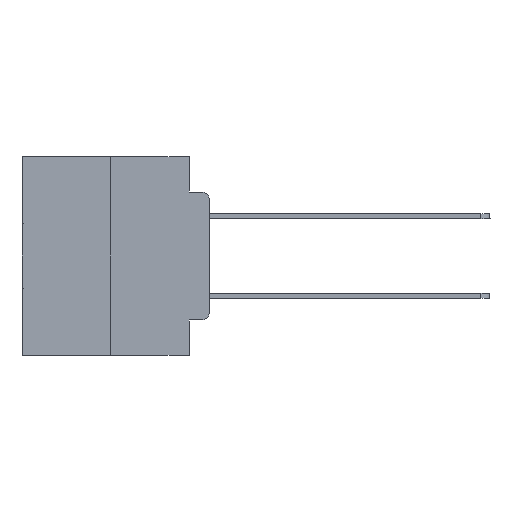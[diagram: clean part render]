
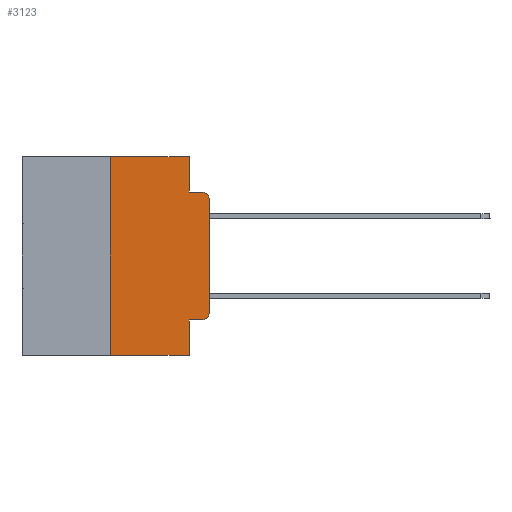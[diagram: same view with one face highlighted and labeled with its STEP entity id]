
A CAD part, left-side view. The second image highlights one B-rep face of the part: STEP entity #3123.
In plain terms, the highlighted planar face has unit normal (-1, 0, 0).
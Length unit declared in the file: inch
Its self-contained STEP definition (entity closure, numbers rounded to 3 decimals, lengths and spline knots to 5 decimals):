
#563 = ORIENTED_EDGE ( 'NONE', *, *, #14449, .T. ) ;
#740 = CARTESIAN_POINT ( 'NONE',  ( 0., 0.25, 0. ) ) ;
#983 = DIRECTION ( 'NONE',  ( 0., 0., -1. ) ) ;
#1638 = CARTESIAN_POINT ( 'NONE',  ( 0., 0.25, 0. ) ) ;
#3033 = LINE ( 'NONE', #27077, #23348 ) ;
#3123 = ADVANCED_FACE ( 'NONE', ( #18397 ), #16786, .F. ) ;
#3356 = CARTESIAN_POINT ( 'NONE',  ( 0., 0.051, -0.0885 ) ) ;
#3423 = CARTESIAN_POINT ( 'NONE',  ( 0., 0.02, -0.3915 ) ) ;
#3511 = DIRECTION ( 'NONE',  ( 0., -1., 0. ) ) ;
#3530 = DIRECTION ( 'NONE',  ( -1., 0., 0. ) ) ;
#3888 = CARTESIAN_POINT ( 'NONE',  ( 0., 0.051, 0. ) ) ;
#4027 = ORIENTED_EDGE ( 'NONE', *, *, #8281, .T. ) ;
#4489 = CARTESIAN_POINT ( 'NONE',  ( 0., 0.051, -0.4115 ) ) ;
#4744 = VECTOR ( 'NONE', #10514, 39.37008 ) ;
#5092 = LINE ( 'NONE', #1638, #18167 ) ;
#5315 = EDGE_CURVE ( 'NONE', #23639, #23531, #3033, .T. ) ;
#5447 = AXIS2_PLACEMENT_3D ( 'NONE', #3423, #3530, #8211 ) ;
#5472 = CARTESIAN_POINT ( 'NONE',  ( 0., 0.02, -0.0885 ) ) ;
#5487 = ORIENTED_EDGE ( 'NONE', *, *, #9553, .F. ) ;
#5528 = CARTESIAN_POINT ( 'NONE',  ( 0., 0., 0. ) ) ;
#5616 = CARTESIAN_POINT ( 'NONE',  ( 0., 0.473, 0. ) ) ;
#5816 = VERTEX_POINT ( 'NONE', #17819 ) ;
#7104 = LINE ( 'NONE', #20192, #11091 ) ;
#7205 = VECTOR ( 'NONE', #11801, 39.37008 ) ;
#8211 = DIRECTION ( 'NONE',  ( 0., 0., -1. ) ) ;
#8272 = EDGE_CURVE ( 'NONE', #5816, #17584, #12028, .T. ) ;
#8281 = EDGE_CURVE ( 'NONE', #17584, #23531, #16006, .T. ) ;
#8688 = VERTEX_POINT ( 'NONE', #740 ) ;
#8963 = ORIENTED_EDGE ( 'NONE', *, *, #17344, .T. ) ;
#9044 = VERTEX_POINT ( 'NONE', #18626 ) ;
#9199 = CARTESIAN_POINT ( 'NONE',  ( 0., 0.473, -0.5 ) ) ;
#9553 = EDGE_CURVE ( 'NONE', #8688, #25416, #18065, .T. ) ;
#10138 = CARTESIAN_POINT ( 'NONE',  ( 0., 0.051, 0. ) ) ;
#10381 = CARTESIAN_POINT ( 'NONE',  ( 0., 0.051, -0.5 ) ) ;
#10427 = DIRECTION ( 'NONE',  ( -1., 0., 0. ) ) ;
#10514 = DIRECTION ( 'NONE',  ( 0., 0., 1. ) ) ;
#11054 = CIRCLE ( 'NONE', #5447, 0.02 ) ;
#11091 = VECTOR ( 'NONE', #26906, 39.37008 ) ;
#11175 = DIRECTION ( 'NONE',  ( 0., 0., 1. ) ) ;
#11345 = EDGE_CURVE ( 'NONE', #25416, #23639, #20902, .T. ) ;
#11752 = EDGE_CURVE ( 'NONE', #22698, #5816, #11054, .T. ) ;
#11801 = DIRECTION ( 'NONE',  ( 0., -1., 0. ) ) ;
#12028 = LINE ( 'NONE', #5528, #4744 ) ;
#12418 = CARTESIAN_POINT ( 'NONE',  ( 0., 0.25, -0.5 ) ) ;
#12474 = LINE ( 'NONE', #4489, #13528 ) ;
#13103 = ORIENTED_EDGE ( 'NONE', *, *, #5315, .F. ) ;
#13157 = ORIENTED_EDGE ( 'NONE', *, *, #13551, .F. ) ;
#13528 = VECTOR ( 'NONE', #20847, 39.37008 ) ;
#13551 = EDGE_CURVE ( 'NONE', #26664, #8688, #5092, .T. ) ;
#14170 = CARTESIAN_POINT ( 'NONE',  ( 0., 0.02, -0.4115 ) ) ;
#14449 = EDGE_CURVE ( 'NONE', #26664, #23641, #16283, .T. ) ;
#15948 = EDGE_CURVE ( 'NONE', #9044, #23641, #7104, .T. ) ;
#16006 = CIRCLE ( 'NONE', #23114, 0.02 ) ;
#16283 = LINE ( 'NONE', #9199, #26847 ) ;
#16722 = ORIENTED_EDGE ( 'NONE', *, *, #11345, .F. ) ;
#16786 = PLANE ( 'NONE',  #23799 ) ;
#17198 = CARTESIAN_POINT ( 'NONE',  ( 0., 0.02, -0.1085 ) ) ;
#17344 = EDGE_CURVE ( 'NONE', #9044, #22698, #12474, .T. ) ;
#17584 = VERTEX_POINT ( 'NONE', #28760 ) ;
#17641 = ORIENTED_EDGE ( 'NONE', *, *, #15948, .F. ) ;
#17819 = CARTESIAN_POINT ( 'NONE',  ( 0., 0., -0.3915 ) ) ;
#18065 = LINE ( 'NONE', #20632, #7205 ) ;
#18167 = VECTOR ( 'NONE', #11175, 39.37008 ) ;
#18397 = FACE_OUTER_BOUND ( 'NONE', #22229, .T. ) ;
#18626 = CARTESIAN_POINT ( 'NONE',  ( 0., 0.051, -0.4115 ) ) ;
#18699 = VECTOR ( 'NONE', #22560, 39.37008 ) ;
#20192 = CARTESIAN_POINT ( 'NONE',  ( 0., 0.051, 0. ) ) ;
#20632 = CARTESIAN_POINT ( 'NONE',  ( 0., 0.473, 0. ) ) ;
#20664 = DIRECTION ( 'NONE',  ( 0., -1., 0. ) ) ;
#20847 = DIRECTION ( 'NONE',  ( 0., -1., 0. ) ) ;
#20902 = LINE ( 'NONE', #3888, #18699 ) ;
#21573 = DIRECTION ( 'NONE',  ( 1., 0., 0. ) ) ;
#22229 = EDGE_LOOP ( 'NONE', ( #29483, #4027, #13103, #16722, #5487, #13157, #563, #17641, #8963, #22524 ) ) ;
#22524 = ORIENTED_EDGE ( 'NONE', *, *, #11752, .T. ) ;
#22560 = DIRECTION ( 'NONE',  ( 0., 0., -1. ) ) ;
#22698 = VERTEX_POINT ( 'NONE', #14170 ) ;
#23114 = AXIS2_PLACEMENT_3D ( 'NONE', #17198, #10427, #28711 ) ;
#23348 = VECTOR ( 'NONE', #3511, 39.37008 ) ;
#23531 = VERTEX_POINT ( 'NONE', #5472 ) ;
#23639 = VERTEX_POINT ( 'NONE', #3356 ) ;
#23641 = VERTEX_POINT ( 'NONE', #10381 ) ;
#23799 = AXIS2_PLACEMENT_3D ( 'NONE', #5616, #21573, #983 ) ;
#25416 = VERTEX_POINT ( 'NONE', #10138 ) ;
#26664 = VERTEX_POINT ( 'NONE', #12418 ) ;
#26847 = VECTOR ( 'NONE', #20664, 39.37008 ) ;
#26906 = DIRECTION ( 'NONE',  ( 0., 0., -1. ) ) ;
#27077 = CARTESIAN_POINT ( 'NONE',  ( 0., 0.051, -0.0885 ) ) ;
#28711 = DIRECTION ( 'NONE',  ( 0., 0., -1. ) ) ;
#28760 = CARTESIAN_POINT ( 'NONE',  ( 0., 0., -0.1085 ) ) ;
#29483 = ORIENTED_EDGE ( 'NONE', *, *, #8272, .T. ) ;
